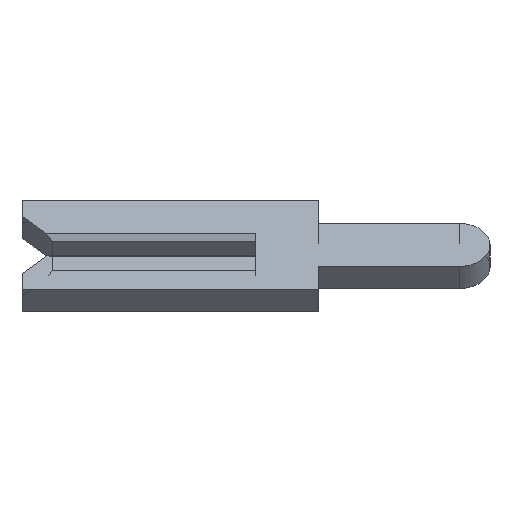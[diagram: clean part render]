
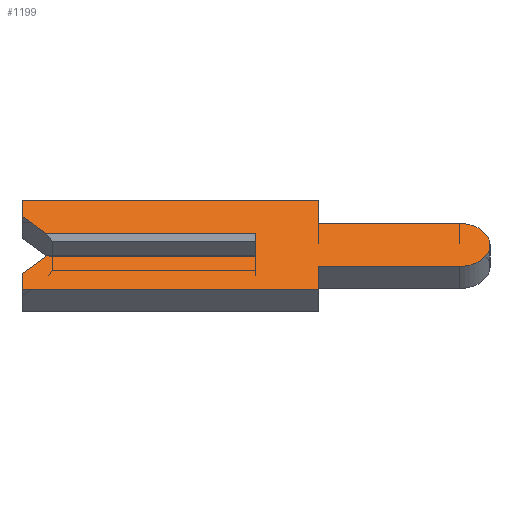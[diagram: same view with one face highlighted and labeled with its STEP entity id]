
A CAD part, left-side view. The second image highlights one B-rep face of the part: STEP entity #1199.
In plain terms, the highlighted face is planar.
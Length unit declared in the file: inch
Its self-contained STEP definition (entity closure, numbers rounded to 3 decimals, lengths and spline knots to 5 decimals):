
#10 = CARTESIAN_POINT ( 'NONE',  ( -0.01, -0.04, -0.0195 ) ) ;
#11 = VECTOR ( 'NONE', #1261, 39.37008 ) ;
#36 = EDGE_CURVE ( 'NONE', #759, #1090, #932, .T. ) ;
#43 = CARTESIAN_POINT ( 'NONE',  ( -0.01, 0.15, -0.026 ) ) ;
#84 = VECTOR ( 'NONE', #460, 39.37008 ) ;
#97 = DIRECTION ( 'NONE',  ( 0., -1., 0. ) ) ;
#182 = CARTESIAN_POINT ( 'NONE',  ( -0.01, 0., 0.01 ) ) ;
#183 = VERTEX_POINT ( 'NONE', #980 ) ;
#227 = CARTESIAN_POINT ( 'NONE',  ( -0.01, 0.134, 0.01 ) ) ;
#233 = VECTOR ( 'NONE', #1873, 39.37008 ) ;
#237 = LINE ( 'NONE', #1217, #1561 ) ;
#240 = EDGE_CURVE ( 'NONE', #479, #2830, #2560, .T. ) ;
#241 = CARTESIAN_POINT ( 'NONE',  ( -0.01, 0.15, -0.026 ) ) ;
#243 = VERTEX_POINT ( 'NONE', #1704 ) ;
#245 = CARTESIAN_POINT ( 'NONE',  ( -0.01, 0., 0.0065 ) ) ;
#266 = CARTESIAN_POINT ( 'NONE',  ( -0.01, -0.04, 0.04 ) ) ;
#267 = LINE ( 'NONE', #428, #1847 ) ;
#316 = EDGE_CURVE ( 'NONE', #1415, #243, #237, .T. ) ;
#365 = EDGE_CURVE ( 'NONE', #2641, #472, #2774, .T. ) ;
#370 = CARTESIAN_POINT ( 'NONE',  ( -0.01, 0., -0.01 ) ) ;
#428 = CARTESIAN_POINT ( 'NONE',  ( -0.01, 0.15, -0.04 ) ) ;
#440 = DIRECTION ( 'NONE',  ( 0., 1., 0. ) ) ;
#460 = DIRECTION ( 'NONE',  ( 0., -0.707, 0.707 ) ) ;
#472 = VERTEX_POINT ( 'NONE', #1532 ) ;
#479 = VERTEX_POINT ( 'NONE', #1283 ) ;
#493 = LINE ( 'NONE', #2646, #1481 ) ;
#497 = DIRECTION ( 'NONE',  ( 1., 0., 0. ) ) ;
#523 = EDGE_CURVE ( 'NONE', #2595, #1415, #2919, .T. ) ;
#553 = DIRECTION ( 'NONE',  ( 0., -1., 0. ) ) ;
#570 = LINE ( 'NONE', #839, #2880 ) ;
#589 = EDGE_LOOP ( 'NONE', ( #591, #2455, #2849, #1147, #2244, #1479, #2718, #2137, #1429, #1537, #963, #1113, #2432, #988 ) ) ;
#591 = ORIENTED_EDGE ( 'NONE', *, *, #803, .T. ) ;
#598 = EDGE_CURVE ( 'NONE', #183, #759, #493, .T. ) ;
#612 = LINE ( 'NONE', #2262, #1699 ) ;
#629 = DIRECTION ( 'NONE',  ( 1., 0., 0. ) ) ;
#636 = DIRECTION ( 'NONE',  ( 0., 1., 0. ) ) ;
#721 = VECTOR ( 'NONE', #1554, 39.37008 ) ;
#759 = VERTEX_POINT ( 'NONE', #370 ) ;
#778 = VERTEX_POINT ( 'NONE', #1992 ) ;
#803 = EDGE_CURVE ( 'NONE', #2294, #1090, #570, .T. ) ;
#839 = CARTESIAN_POINT ( 'NONE',  ( -0.01, 0.15, 0.01 ) ) ;
#932 = LINE ( 'NONE', #245, #1654 ) ;
#963 = ORIENTED_EDGE ( 'NONE', *, *, #523, .F. ) ;
#980 = CARTESIAN_POINT ( 'NONE',  ( -0.01, 0.134, -0.01 ) ) ;
#988 = ORIENTED_EDGE ( 'NONE', *, *, #1419, .F. ) ;
#1000 = CIRCLE ( 'NONE', #1444, 0.0195 ) ;
#1002 = FACE_OUTER_BOUND ( 'NONE', #589, .T. ) ;
#1039 = VECTOR ( 'NONE', #2853, 39.37008 ) ;
#1044 = EDGE_CURVE ( 'NONE', #2684, #2641, #1064, .T. ) ;
#1064 = LINE ( 'NONE', #2915, #2381 ) ;
#1076 = CARTESIAN_POINT ( 'NONE',  ( -0.01, -0.04, 0.0195 ) ) ;
#1090 = VERTEX_POINT ( 'NONE', #182 ) ;
#1099 = DIRECTION ( 'NONE',  ( 0., -1., 0. ) ) ;
#1107 = CARTESIAN_POINT ( 'NONE',  ( -0.01, -0.1305, 0. ) ) ;
#1113 = ORIENTED_EDGE ( 'NONE', *, *, #1458, .F. ) ;
#1147 = ORIENTED_EDGE ( 'NONE', *, *, #2136, .F. ) ;
#1150 = LINE ( 'NONE', #2731, #721 ) ;
#1199 = ADVANCED_FACE ( 'NONE', ( #1002 ), #2890, .F. ) ;
#1200 = DIRECTION ( 'NONE',  ( 0., 0., 1. ) ) ;
#1217 = CARTESIAN_POINT ( 'NONE',  ( -0.01, -0.04, 0.0195 ) ) ;
#1261 = DIRECTION ( 'NONE',  ( 0., 0., -1. ) ) ;
#1283 = CARTESIAN_POINT ( 'NONE',  ( -0.01, 0.15, -0.04 ) ) ;
#1415 = VERTEX_POINT ( 'NONE', #1076 ) ;
#1419 = EDGE_CURVE ( 'NONE', #2294, #1608, #612, .T. ) ;
#1429 = ORIENTED_EDGE ( 'NONE', *, *, #2551, .F. ) ;
#1444 = AXIS2_PLACEMENT_3D ( 'NONE', #1651, #497, #2553 ) ;
#1458 = EDGE_CURVE ( 'NONE', #778, #2595, #1150, .T. ) ;
#1479 = ORIENTED_EDGE ( 'NONE', *, *, #1931, .F. ) ;
#1481 = VECTOR ( 'NONE', #97, 39.37008 ) ;
#1518 = AXIS2_PLACEMENT_3D ( 'NONE', #1107, #629, #1811 ) ;
#1532 = CARTESIAN_POINT ( 'NONE',  ( -0.01, -0.04, -0.04 ) ) ;
#1537 = ORIENTED_EDGE ( 'NONE', *, *, #316, .F. ) ;
#1554 = DIRECTION ( 'NONE',  ( 0., -1., 0. ) ) ;
#1561 = VECTOR ( 'NONE', #553, 39.37008 ) ;
#1608 = VERTEX_POINT ( 'NONE', #2544 ) ;
#1651 = CARTESIAN_POINT ( 'NONE',  ( -0.01, -0.1305, 0. ) ) ;
#1654 = VECTOR ( 'NONE', #1200, 39.37008 ) ;
#1699 = VECTOR ( 'NONE', #2474, 39.37008 ) ;
#1704 = CARTESIAN_POINT ( 'NONE',  ( -0.01, -0.1305, 0.0195 ) ) ;
#1811 = DIRECTION ( 'NONE',  ( 0., 0., -1. ) ) ;
#1847 = VECTOR ( 'NONE', #440, 39.37008 ) ;
#1855 = CARTESIAN_POINT ( 'NONE',  ( -0.01, 0.1305, -0.0065 ) ) ;
#1873 = DIRECTION ( 'NONE',  ( 0., 0., 1. ) ) ;
#1879 = VECTOR ( 'NONE', #1928, 39.37008 ) ;
#1928 = DIRECTION ( 'NONE',  ( 0., 0., 1. ) ) ;
#1931 = EDGE_CURVE ( 'NONE', #472, #479, #267, .T. ) ;
#1992 = CARTESIAN_POINT ( 'NONE',  ( -0.01, 0.15, 0.04 ) ) ;
#2100 = CARTESIAN_POINT ( 'NONE',  ( -0.01, -0.1305, -0.0195 ) ) ;
#2119 = CARTESIAN_POINT ( 'NONE',  ( -0.01, 0.15, 0.026 ) ) ;
#2136 = EDGE_CURVE ( 'NONE', #2830, #183, #2488, .T. ) ;
#2137 = ORIENTED_EDGE ( 'NONE', *, *, #1044, .F. ) ;
#2171 = CARTESIAN_POINT ( 'NONE',  ( -0.01, -0.04, 0.04 ) ) ;
#2244 = ORIENTED_EDGE ( 'NONE', *, *, #240, .F. ) ;
#2262 = CARTESIAN_POINT ( 'NONE',  ( -0.01, 0.1305, 0.0065 ) ) ;
#2294 = VERTEX_POINT ( 'NONE', #227 ) ;
#2381 = VECTOR ( 'NONE', #636, 39.37008 ) ;
#2402 = CARTESIAN_POINT ( 'NONE',  ( -0.01, -0.04, -0.04 ) ) ;
#2432 = ORIENTED_EDGE ( 'NONE', *, *, #2899, .F. ) ;
#2455 = ORIENTED_EDGE ( 'NONE', *, *, #36, .F. ) ;
#2474 = DIRECTION ( 'NONE',  ( 0., 0.707, 0.707 ) ) ;
#2488 = LINE ( 'NONE', #1855, #84 ) ;
#2544 = CARTESIAN_POINT ( 'NONE',  ( -0.01, 0.15, 0.026 ) ) ;
#2551 = EDGE_CURVE ( 'NONE', #243, #2684, #1000, .T. ) ;
#2553 = DIRECTION ( 'NONE',  ( 0., 0., -1. ) ) ;
#2558 = LINE ( 'NONE', #2119, #233 ) ;
#2560 = LINE ( 'NONE', #43, #1879 ) ;
#2595 = VERTEX_POINT ( 'NONE', #266 ) ;
#2641 = VERTEX_POINT ( 'NONE', #10 ) ;
#2646 = CARTESIAN_POINT ( 'NONE',  ( -0.01, -0.1305, -0.01 ) ) ;
#2684 = VERTEX_POINT ( 'NONE', #2100 ) ;
#2718 = ORIENTED_EDGE ( 'NONE', *, *, #365, .F. ) ;
#2731 = CARTESIAN_POINT ( 'NONE',  ( -0.01, 0.15, 0.04 ) ) ;
#2774 = LINE ( 'NONE', #2402, #1039 ) ;
#2830 = VERTEX_POINT ( 'NONE', #241 ) ;
#2849 = ORIENTED_EDGE ( 'NONE', *, *, #598, .F. ) ;
#2853 = DIRECTION ( 'NONE',  ( 0., 0., -1. ) ) ;
#2880 = VECTOR ( 'NONE', #1099, 39.37008 ) ;
#2890 = PLANE ( 'NONE',  #1518 ) ;
#2899 = EDGE_CURVE ( 'NONE', #1608, #778, #2558, .T. ) ;
#2915 = CARTESIAN_POINT ( 'NONE',  ( -0.01, -0.04, -0.0195 ) ) ;
#2919 = LINE ( 'NONE', #2171, #11 ) ;
